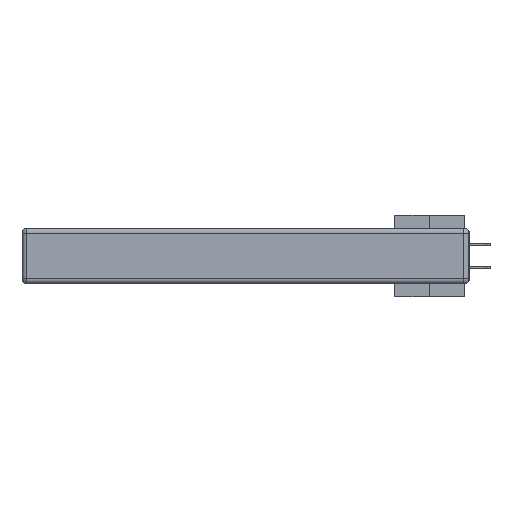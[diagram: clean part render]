
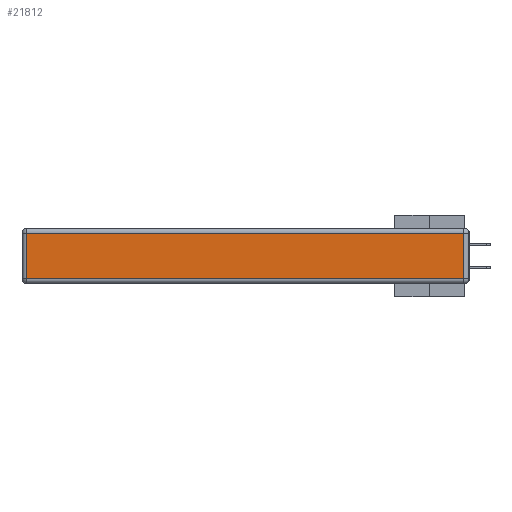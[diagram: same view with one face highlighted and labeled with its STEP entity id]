
A CAD part, left-side view. The second image highlights one B-rep face of the part: STEP entity #21812.
In plain terms, the highlighted planar face has unit normal (-1, 0, 0).
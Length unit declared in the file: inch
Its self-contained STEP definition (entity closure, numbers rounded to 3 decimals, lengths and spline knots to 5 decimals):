
#1772 = CARTESIAN_POINT ( 'NONE',  ( 0., 0.03, -0.03 ) ) ;
#4210 = EDGE_CURVE ( 'NONE', #33637, #5952, #11179, .T. ) ;
#4915 = CARTESIAN_POINT ( 'NONE',  ( 0., 2.72, -0.343 ) ) ;
#5852 = ORIENTED_EDGE ( 'NONE', *, *, #4210, .T. ) ;
#5952 = VERTEX_POINT ( 'NONE', #20678 ) ;
#7359 = CARTESIAN_POINT ( 'NONE',  ( 0., 0.03, -0.343 ) ) ;
#7635 = ORIENTED_EDGE ( 'NONE', *, *, #9565, .T. ) ;
#9565 = EDGE_CURVE ( 'NONE', #17112, #33637, #26512, .T. ) ;
#10878 = CARTESIAN_POINT ( 'NONE',  ( 0., 0.03, -0.313 ) ) ;
#11179 = LINE ( 'NONE', #22404, #26962 ) ;
#15526 = DIRECTION ( 'NONE',  ( 0., 1., 0. ) ) ;
#17112 = VERTEX_POINT ( 'NONE', #10878 ) ;
#18161 = ORIENTED_EDGE ( 'NONE', *, *, #28519, .T. ) ;
#18250 = CARTESIAN_POINT ( 'NONE',  ( 0., 0., -0.313 ) ) ;
#20444 = ORIENTED_EDGE ( 'NONE', *, *, #40985, .T. ) ;
#20451 = CARTESIAN_POINT ( 'NONE',  ( 0., 0., -0.343 ) ) ;
#20678 = CARTESIAN_POINT ( 'NONE',  ( 0., 2.72, -0.03 ) ) ;
#21788 = DIRECTION ( 'NONE',  ( 0., -1., 0. ) ) ;
#21812 = ADVANCED_FACE ( 'NONE', ( #36768 ), #41386, .T. ) ;
#21956 = VECTOR ( 'NONE', #21788, 39.37008 ) ;
#22404 = CARTESIAN_POINT ( 'NONE',  ( 0., 2.75, -0.03 ) ) ;
#25543 = VERTEX_POINT ( 'NONE', #41074 ) ;
#26512 = LINE ( 'NONE', #7359, #44001 ) ;
#26962 = VECTOR ( 'NONE', #15526, 39.37008 ) ;
#28294 = LINE ( 'NONE', #4915, #39786 ) ;
#28519 = EDGE_CURVE ( 'NONE', #25543, #17112, #31796, .T. ) ;
#31542 = AXIS2_PLACEMENT_3D ( 'NONE', #20451, #34675, #34813 ) ;
#31796 = LINE ( 'NONE', #18250, #21956 ) ;
#33303 = DIRECTION ( 'NONE',  ( 0., 0., -1. ) ) ;
#33637 = VERTEX_POINT ( 'NONE', #1772 ) ;
#34675 = DIRECTION ( 'NONE',  ( -1., 0., 0. ) ) ;
#34813 = DIRECTION ( 'NONE',  ( 0., 0., 1. ) ) ;
#36768 = FACE_OUTER_BOUND ( 'NONE', #43421, .T. ) ;
#39698 = DIRECTION ( 'NONE',  ( 0., 0., 1. ) ) ;
#39786 = VECTOR ( 'NONE', #33303, 39.37008 ) ;
#40985 = EDGE_CURVE ( 'NONE', #5952, #25543, #28294, .T. ) ;
#41074 = CARTESIAN_POINT ( 'NONE',  ( 0., 2.72, -0.313 ) ) ;
#41386 = PLANE ( 'NONE',  #31542 ) ;
#43421 = EDGE_LOOP ( 'NONE', ( #18161, #7635, #5852, #20444 ) ) ;
#44001 = VECTOR ( 'NONE', #39698, 39.37008 ) ;
